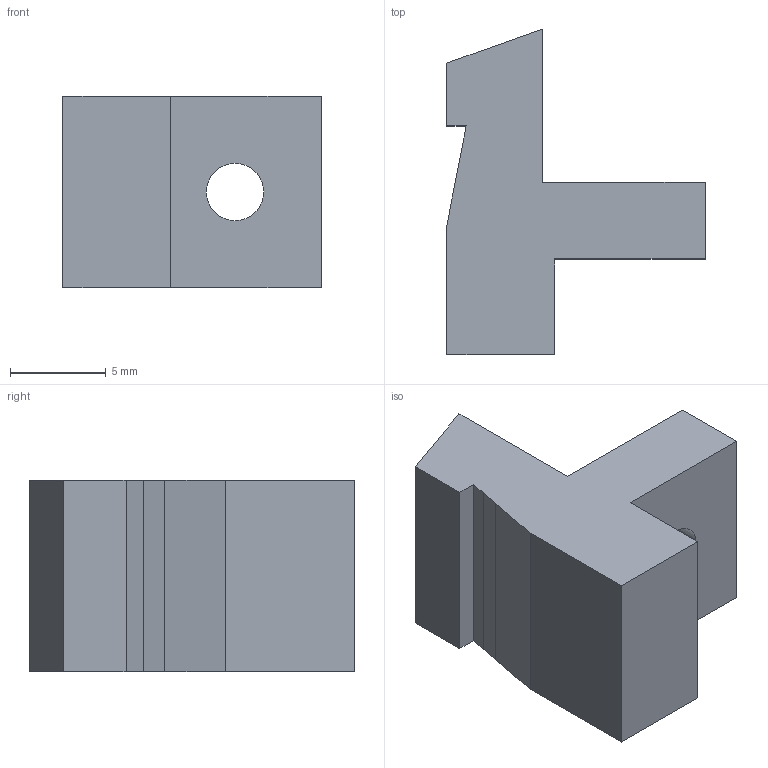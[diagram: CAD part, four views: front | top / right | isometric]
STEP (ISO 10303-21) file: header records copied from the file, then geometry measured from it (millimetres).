
FILE_DESCRIPTION(/* description */ (''),/* implementation_level */ '2;1');
FILE_NAME(/* author */ (''),/* organization */ (''),/* preprocessor_version */ 'ST-DEVELOPER v18.1',/* originating_system */ 'Autodesk Translation Framework v9.3.0.1241',/* authorisation */ '');
FILE_SCHEMA (('AUTOMOTIVE_DESIGN { 1 0 10303 214 3 1 1 }'));
Length unit declared in the file: inch
Products named in the file (1): Beretta_Feedramp_MOD9v2
Bounding box: 13.5 x 17.02 x 10 mm (x, y, z)
Volume: 1096.4 mm3; surface area: 854.8 mm2
Topology: 1 solids, 1 shells, 18 faces, 47 edges, 31 vertices
Faces by surface type: plane 16, cone 1, cylinder 1
Full cylindrical faces by diameter (mm): 3 x1
Entity records: 585 total; most frequent: CARTESIAN_POINT 97, ORIENTED_EDGE 94, DIRECTION 88, EDGE_CURVE 47, LINE 44, VECTOR 44, VERTEX_POINT 31, AXIS2_PLACEMENT_3D 22
